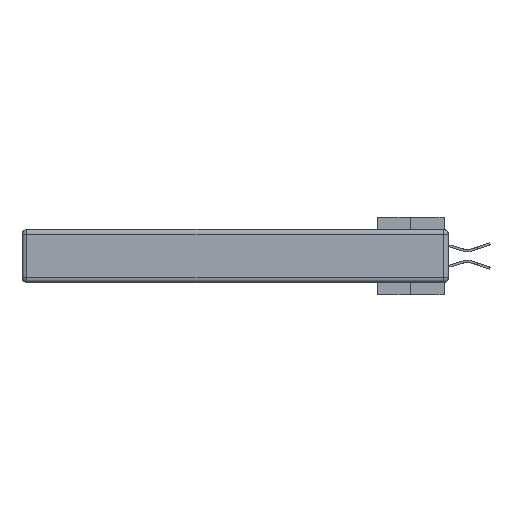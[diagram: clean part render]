
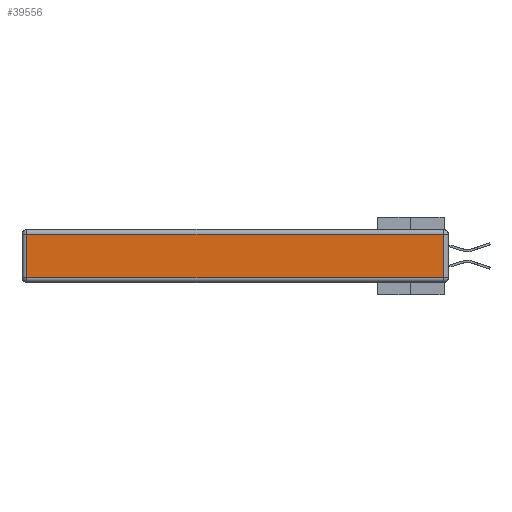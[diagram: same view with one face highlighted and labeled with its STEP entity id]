
A CAD part, left-side view. The second image highlights one B-rep face of the part: STEP entity #39556.
In plain terms, the highlighted planar face has unit normal (-1, 0, 0).
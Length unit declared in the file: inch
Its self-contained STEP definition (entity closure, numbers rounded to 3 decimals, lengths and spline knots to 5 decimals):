
#95 = VECTOR ( 'NONE', #36299, 39.37008 ) ;
#892 = CARTESIAN_POINT ( 'NONE',  ( 0., 2.72, -0.313 ) ) ;
#2180 = CARTESIAN_POINT ( 'NONE',  ( 0., 2.72, -0.343 ) ) ;
#3576 = DIRECTION ( 'NONE',  ( -1., 0., 0. ) ) ;
#4010 = VERTEX_POINT ( 'NONE', #892 ) ;
#4371 = LINE ( 'NONE', #2180, #31605 ) ;
#7581 = CARTESIAN_POINT ( 'NONE',  ( 0., 0.03, -0.313 ) ) ;
#9411 = FACE_OUTER_BOUND ( 'NONE', #29271, .T. ) ;
#10318 = VERTEX_POINT ( 'NONE', #14152 ) ;
#11063 = DIRECTION ( 'NONE',  ( 0., 1., 0. ) ) ;
#13297 = VERTEX_POINT ( 'NONE', #7581 ) ;
#13816 = CARTESIAN_POINT ( 'NONE',  ( 0., 2.72, -0.03 ) ) ;
#13936 = VECTOR ( 'NONE', #11063, 39.37008 ) ;
#14152 = CARTESIAN_POINT ( 'NONE',  ( 0., 0.03, -0.03 ) ) ;
#16075 = EDGE_CURVE ( 'NONE', #4010, #13297, #22401, .T. ) ;
#16807 = CARTESIAN_POINT ( 'NONE',  ( 0., 2.75, -0.03 ) ) ;
#20091 = ORIENTED_EDGE ( 'NONE', *, *, #37859, .T. ) ;
#20997 = CARTESIAN_POINT ( 'NONE',  ( 0., 0., -0.343 ) ) ;
#22401 = LINE ( 'NONE', #33203, #95 ) ;
#23121 = LINE ( 'NONE', #43040, #36989 ) ;
#25026 = DIRECTION ( 'NONE',  ( 0., 0., 1. ) ) ;
#26916 = ORIENTED_EDGE ( 'NONE', *, *, #30874, .T. ) ;
#28727 = AXIS2_PLACEMENT_3D ( 'NONE', #20997, #3576, #25026 ) ;
#29271 = EDGE_LOOP ( 'NONE', ( #41556, #20091, #40759, #26916 ) ) ;
#30874 = EDGE_CURVE ( 'NONE', #32956, #4010, #4371, .T. ) ;
#31605 = VECTOR ( 'NONE', #45307, 39.37008 ) ;
#31832 = PLANE ( 'NONE',  #28727 ) ;
#32956 = VERTEX_POINT ( 'NONE', #13816 ) ;
#33203 = CARTESIAN_POINT ( 'NONE',  ( 0., 0., -0.313 ) ) ;
#34237 = EDGE_CURVE ( 'NONE', #10318, #32956, #41124, .T. ) ;
#36299 = DIRECTION ( 'NONE',  ( 0., -1., 0. ) ) ;
#36566 = DIRECTION ( 'NONE',  ( 0., 0., 1. ) ) ;
#36989 = VECTOR ( 'NONE', #36566, 39.37008 ) ;
#37859 = EDGE_CURVE ( 'NONE', #13297, #10318, #23121, .T. ) ;
#39556 = ADVANCED_FACE ( 'NONE', ( #9411 ), #31832, .T. ) ;
#40759 = ORIENTED_EDGE ( 'NONE', *, *, #34237, .T. ) ;
#41124 = LINE ( 'NONE', #16807, #13936 ) ;
#41556 = ORIENTED_EDGE ( 'NONE', *, *, #16075, .T. ) ;
#43040 = CARTESIAN_POINT ( 'NONE',  ( 0., 0.03, -0.343 ) ) ;
#45307 = DIRECTION ( 'NONE',  ( 0., 0., -1. ) ) ;
